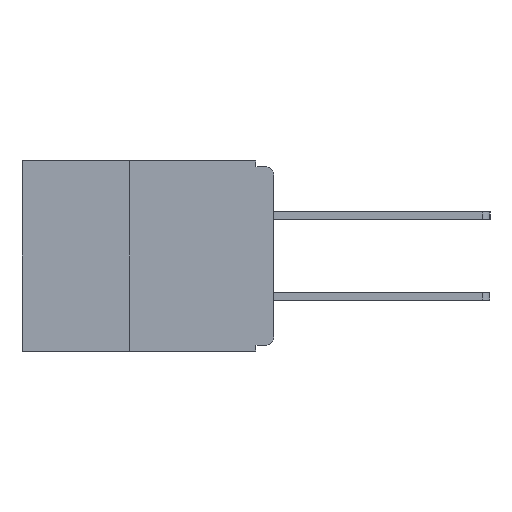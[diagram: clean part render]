
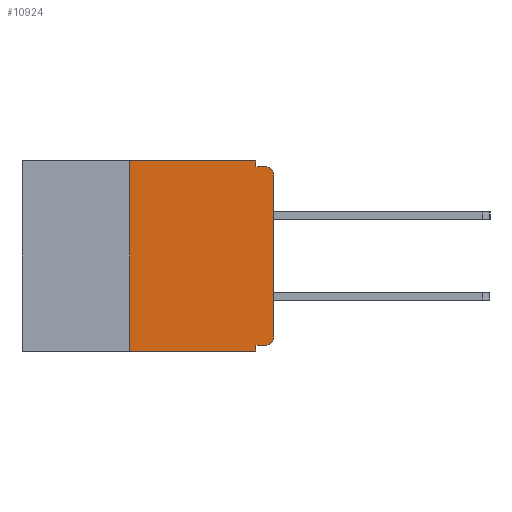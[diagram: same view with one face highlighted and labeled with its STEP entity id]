
A CAD part, left-side view. The second image highlights one B-rep face of the part: STEP entity #10924.
In plain terms, the highlighted planar face has unit normal (-1, 0, 0).
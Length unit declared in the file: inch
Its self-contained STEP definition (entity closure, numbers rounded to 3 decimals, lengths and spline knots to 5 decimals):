
#252 = VERTEX_POINT ( 'NONE', #12757 ) ;
#258 = CARTESIAN_POINT ( 'NONE',  ( 0., 0.25, -0.33 ) ) ;
#730 = DIRECTION ( 'NONE',  ( 0., 0., 1. ) ) ;
#878 = DIRECTION ( 'NONE',  ( 0., -1., 0. ) ) ;
#1305 = EDGE_CURVE ( 'NONE', #4099, #8507, #5201, .T. ) ;
#1438 = AXIS2_PLACEMENT_3D ( 'NONE', #5398, #13830, #6601 ) ;
#1475 = CARTESIAN_POINT ( 'NONE',  ( 0., 0.031, 0. ) ) ;
#1698 = EDGE_CURVE ( 'NONE', #1997, #11515, #3058, .T. ) ;
#1699 = CIRCLE ( 'NONE', #1438, 0.015 ) ;
#1890 = LINE ( 'NONE', #6292, #4755 ) ;
#1963 = CARTESIAN_POINT ( 'NONE',  ( 0., 0.031, -0.32 ) ) ;
#1979 = EDGE_CURVE ( 'NONE', #12457, #13856, #5358, .T. ) ;
#1997 = VERTEX_POINT ( 'NONE', #4618 ) ;
#2255 = EDGE_CURVE ( 'NONE', #6131, #4099, #4784, .T. ) ;
#2412 = CARTESIAN_POINT ( 'NONE',  ( 0., 0., -0.01 ) ) ;
#3058 = LINE ( 'NONE', #2412, #15165 ) ;
#3502 = LINE ( 'NONE', #12113, #10369 ) ;
#3539 = LINE ( 'NONE', #5601, #6421 ) ;
#4099 = VERTEX_POINT ( 'NONE', #14052 ) ;
#4291 = DIRECTION ( 'NONE',  ( 0., 0., -1. ) ) ;
#4412 = CARTESIAN_POINT ( 'NONE',  ( 0., 0.031, -0.33 ) ) ;
#4618 = CARTESIAN_POINT ( 'NONE',  ( 0., 0.031, -0.01 ) ) ;
#4755 = VECTOR ( 'NONE', #7488, 39.37008 ) ;
#4784 = LINE ( 'NONE', #258, #10867 ) ;
#5018 = EDGE_CURVE ( 'NONE', #10566, #6032, #10407, .T. ) ;
#5046 = VECTOR ( 'NONE', #8009, 39.37008 ) ;
#5171 = DIRECTION ( 'NONE',  ( 0., 0., -1. ) ) ;
#5201 = LINE ( 'NONE', #13125, #11265 ) ;
#5358 = LINE ( 'NONE', #4412, #14629 ) ;
#5398 = CARTESIAN_POINT ( 'NONE',  ( 0., 0.015, -0.025 ) ) ;
#5523 = ORIENTED_EDGE ( 'NONE', *, *, #1305, .F. ) ;
#5601 = CARTESIAN_POINT ( 'NONE',  ( 0., 0.031, 0. ) ) ;
#5719 = ORIENTED_EDGE ( 'NONE', *, *, #12429, .F. ) ;
#6032 = VERTEX_POINT ( 'NONE', #12320 ) ;
#6131 = VERTEX_POINT ( 'NONE', #8678 ) ;
#6292 = CARTESIAN_POINT ( 'NONE',  ( 0., 0.437, -0.33 ) ) ;
#6327 = CARTESIAN_POINT ( 'NONE',  ( 0., 0.437, 0. ) ) ;
#6421 = VECTOR ( 'NONE', #7964, 39.37008 ) ;
#6601 = DIRECTION ( 'NONE',  ( 0., 0., -1. ) ) ;
#6726 = EDGE_CURVE ( 'NONE', #6032, #252, #13901, .T. ) ;
#7115 = CARTESIAN_POINT ( 'NONE',  ( 0., 0., 0. ) ) ;
#7293 = ORIENTED_EDGE ( 'NONE', *, *, #10300, .T. ) ;
#7488 = DIRECTION ( 'NONE',  ( 0., -1., 0. ) ) ;
#7627 = ORIENTED_EDGE ( 'NONE', *, *, #9836, .T. ) ;
#7964 = DIRECTION ( 'NONE',  ( 0., 0., -1. ) ) ;
#7988 = ORIENTED_EDGE ( 'NONE', *, *, #1698, .F. ) ;
#8009 = DIRECTION ( 'NONE',  ( 0., 0., 1. ) ) ;
#8507 = VERTEX_POINT ( 'NONE', #1475 ) ;
#8678 = CARTESIAN_POINT ( 'NONE',  ( 0., 0.25, -0.33 ) ) ;
#9137 = CARTESIAN_POINT ( 'NONE',  ( 0., 0.015, -0.32 ) ) ;
#9652 = ORIENTED_EDGE ( 'NONE', *, *, #6726, .T. ) ;
#9732 = DIRECTION ( 'NONE',  ( 0., -1., 0. ) ) ;
#9836 = EDGE_CURVE ( 'NONE', #252, #11515, #1699, .T. ) ;
#9910 = CARTESIAN_POINT ( 'NONE',  ( 0., 0.015, -0.01 ) ) ;
#9987 = PLANE ( 'NONE',  #10291 ) ;
#10003 = AXIS2_PLACEMENT_3D ( 'NONE', #15411, #15378, #15307 ) ;
#10291 = AXIS2_PLACEMENT_3D ( 'NONE', #6327, #12430, #5171 ) ;
#10300 = EDGE_CURVE ( 'NONE', #6131, #13856, #1890, .T. ) ;
#10369 = VECTOR ( 'NONE', #14516, 39.37008 ) ;
#10407 = CIRCLE ( 'NONE', #10003, 0.015 ) ;
#10566 = VERTEX_POINT ( 'NONE', #9137 ) ;
#10867 = VECTOR ( 'NONE', #730, 39.37008 ) ;
#10924 = ADVANCED_FACE ( 'NONE', ( #15289 ), #9987, .F. ) ;
#11126 = ORIENTED_EDGE ( 'NONE', *, *, #5018, .T. ) ;
#11265 = VECTOR ( 'NONE', #878, 39.37008 ) ;
#11515 = VERTEX_POINT ( 'NONE', #9910 ) ;
#11680 = ORIENTED_EDGE ( 'NONE', *, *, #1979, .F. ) ;
#12113 = CARTESIAN_POINT ( 'NONE',  ( 0., 0., -0.32 ) ) ;
#12320 = CARTESIAN_POINT ( 'NONE',  ( 0., 0., -0.305 ) ) ;
#12429 = EDGE_CURVE ( 'NONE', #8507, #1997, #3539, .T. ) ;
#12430 = DIRECTION ( 'NONE',  ( 1., 0., 0. ) ) ;
#12457 = VERTEX_POINT ( 'NONE', #1963 ) ;
#12757 = CARTESIAN_POINT ( 'NONE',  ( 0., 0., -0.025 ) ) ;
#12806 = ORIENTED_EDGE ( 'NONE', *, *, #14374, .F. ) ;
#13125 = CARTESIAN_POINT ( 'NONE',  ( 0., 0.437, 0. ) ) ;
#13405 = CARTESIAN_POINT ( 'NONE',  ( 0., 0.031, -0.33 ) ) ;
#13830 = DIRECTION ( 'NONE',  ( -1., 0., 0. ) ) ;
#13856 = VERTEX_POINT ( 'NONE', #13405 ) ;
#13901 = LINE ( 'NONE', #7115, #5046 ) ;
#14052 = CARTESIAN_POINT ( 'NONE',  ( 0., 0.25, 0. ) ) ;
#14374 = EDGE_CURVE ( 'NONE', #10566, #12457, #3502, .T. ) ;
#14516 = DIRECTION ( 'NONE',  ( 0., 1., 0. ) ) ;
#14629 = VECTOR ( 'NONE', #4291, 39.37008 ) ;
#14666 = EDGE_LOOP ( 'NONE', ( #9652, #7627, #7988, #5719, #5523, #14669, #7293, #11680, #12806, #11126 ) ) ;
#14669 = ORIENTED_EDGE ( 'NONE', *, *, #2255, .F. ) ;
#15165 = VECTOR ( 'NONE', #9732, 39.37008 ) ;
#15289 = FACE_OUTER_BOUND ( 'NONE', #14666, .T. ) ;
#15307 = DIRECTION ( 'NONE',  ( 0., 0., -1. ) ) ;
#15378 = DIRECTION ( 'NONE',  ( -1., 0., 0. ) ) ;
#15411 = CARTESIAN_POINT ( 'NONE',  ( 0., 0.015, -0.305 ) ) ;
